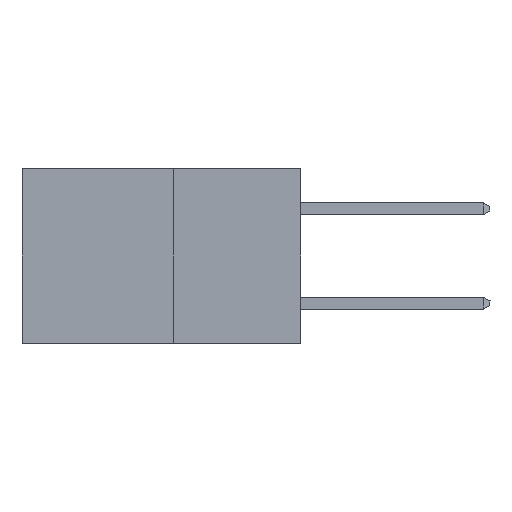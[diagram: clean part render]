
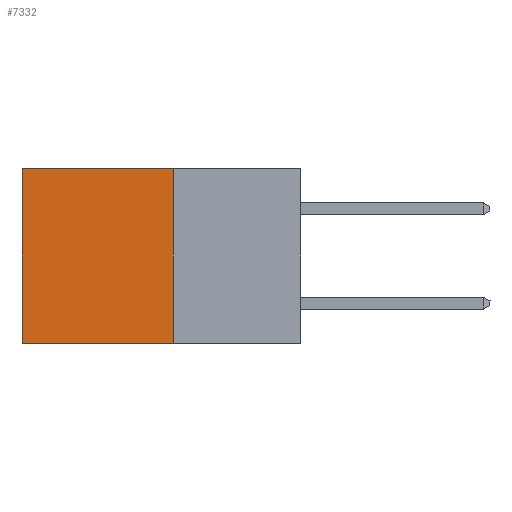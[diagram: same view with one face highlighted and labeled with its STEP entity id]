
A CAD part, left-side view. The second image highlights one B-rep face of the part: STEP entity #7332.
In plain terms, the highlighted planar face has unit normal (-1, 0, 0).
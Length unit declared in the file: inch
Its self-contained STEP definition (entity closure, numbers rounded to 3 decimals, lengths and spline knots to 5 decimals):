
#198 = EDGE_CURVE ( 'NONE', #10233, #4998, #4316, .T. ) ;
#204 = VERTEX_POINT ( 'NONE', #3756 ) ;
#762 = ORIENTED_EDGE ( 'NONE', *, *, #198, .F. ) ;
#1181 = ORIENTED_EDGE ( 'NONE', *, *, #5402, .F. ) ;
#1501 = CARTESIAN_POINT ( 'NONE',  ( 0.277, 0.27, -0.37 ) ) ;
#1569 = LINE ( 'NONE', #8165, #10957 ) ;
#1592 = ORIENTED_EDGE ( 'NONE', *, *, #1999, .T. ) ;
#1920 = VECTOR ( 'NONE', #5970, 39.37008 ) ;
#1999 = EDGE_CURVE ( 'NONE', #204, #8011, #7128, .T. ) ;
#2412 = EDGE_LOOP ( 'NONE', ( #1592, #1181, #762, #3025 ) ) ;
#2497 = CARTESIAN_POINT ( 'NONE',  ( 0.277, 0.59, -0.37 ) ) ;
#3025 = ORIENTED_EDGE ( 'NONE', *, *, #6982, .T. ) ;
#3710 = CARTESIAN_POINT ( 'NONE',  ( 0.277, 0.27, -0.37 ) ) ;
#3756 = CARTESIAN_POINT ( 'NONE',  ( 0.277, 0.59, 0. ) ) ;
#3772 = DIRECTION ( 'NONE',  ( 0., 0., -1. ) ) ;
#3781 = DIRECTION ( 'NONE',  ( 1., 0., 0. ) ) ;
#4316 = LINE ( 'NONE', #1501, #1920 ) ;
#4759 = VECTOR ( 'NONE', #5310, 39.37008 ) ;
#4998 = VERTEX_POINT ( 'NONE', #10918 ) ;
#5310 = DIRECTION ( 'NONE',  ( 0., 0., -1. ) ) ;
#5402 = EDGE_CURVE ( 'NONE', #4998, #8011, #8942, .T. ) ;
#5970 = DIRECTION ( 'NONE',  ( 0., 0., -1. ) ) ;
#6561 = PLANE ( 'NONE',  #7396 ) ;
#6631 = VECTOR ( 'NONE', #8065, 39.37008 ) ;
#6682 = CARTESIAN_POINT ( 'NONE',  ( 0.277, 0.59, -0.37 ) ) ;
#6982 = EDGE_CURVE ( 'NONE', #10233, #204, #1569, .T. ) ;
#7128 = LINE ( 'NONE', #6682, #4759 ) ;
#7332 = ADVANCED_FACE ( 'NONE', ( #9702 ), #6561, .F. ) ;
#7396 = AXIS2_PLACEMENT_3D ( 'NONE', #3710, #3781, #3772 ) ;
#8011 = VERTEX_POINT ( 'NONE', #2497 ) ;
#8065 = DIRECTION ( 'NONE',  ( 0., 1., 0. ) ) ;
#8092 = CARTESIAN_POINT ( 'NONE',  ( 0.277, 0.27, -0.37 ) ) ;
#8131 = DIRECTION ( 'NONE',  ( 0., 1., 0. ) ) ;
#8165 = CARTESIAN_POINT ( 'NONE',  ( 0.277, 0.27, 0. ) ) ;
#8506 = CARTESIAN_POINT ( 'NONE',  ( 0.277, 0.27, 0. ) ) ;
#8942 = LINE ( 'NONE', #8092, #6631 ) ;
#9702 = FACE_OUTER_BOUND ( 'NONE', #2412, .T. ) ;
#10233 = VERTEX_POINT ( 'NONE', #8506 ) ;
#10918 = CARTESIAN_POINT ( 'NONE',  ( 0.277, 0.27, -0.37 ) ) ;
#10957 = VECTOR ( 'NONE', #8131, 39.37008 ) ;
